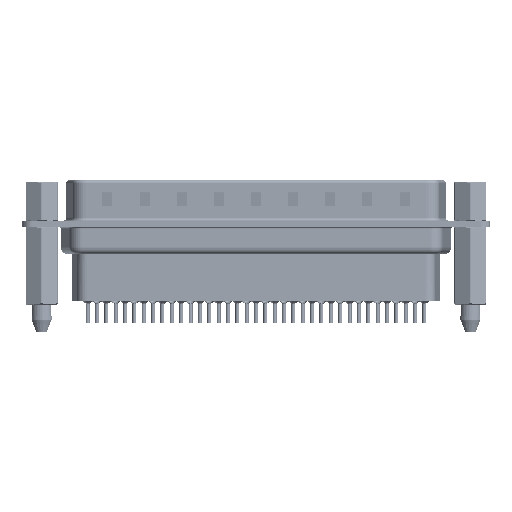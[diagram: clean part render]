
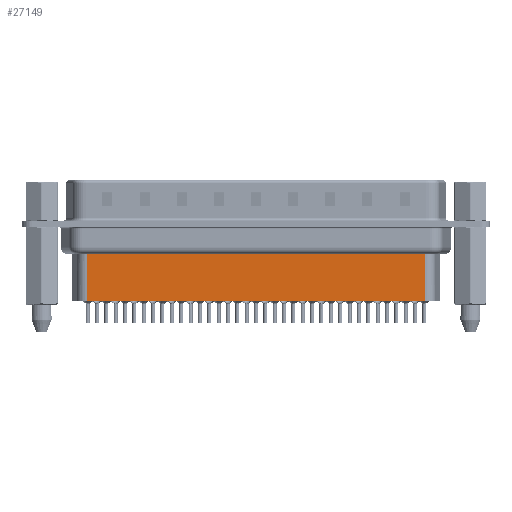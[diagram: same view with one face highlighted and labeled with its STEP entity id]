
A CAD part, front view. The second image highlights one B-rep face of the part: STEP entity #27149.
In plain terms, the highlighted planar face has unit normal (0, -1, 0).
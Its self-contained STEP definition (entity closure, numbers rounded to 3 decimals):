
#1149 = VECTOR ( 'NONE', #17048, 1000. ) ;
#1164 = EDGE_CURVE ( 'NONE', #26078, #18752, #14244, .T. ) ;
#1530 = CARTESIAN_POINT ( 'NONE',  ( 6.459, -3.5, -4.097 ) ) ;
#1653 = DIRECTION ( 'NONE',  ( -1., 0., 0. ) ) ;
#2057 = LINE ( 'NONE', #8477, #1149 ) ;
#3252 = CARTESIAN_POINT ( 'NONE',  ( 6.706, -3.5, -3.1 ) ) ;
#5884 = ORIENTED_EDGE ( 'NONE', *, *, #16960, .F. ) ;
#6689 = VECTOR ( 'NONE', #30666, 1000. ) ;
#8477 = CARTESIAN_POINT ( 'NONE',  ( 6.706, -3.5, -11.45 ) ) ;
#9018 = PLANE ( 'NONE',  #17963 ) ;
#9778 = VECTOR ( 'NONE', #1653, 1000. ) ;
#11886 = DIRECTION ( 'NONE',  ( 0., -1., 0. ) ) ;
#11914 = CARTESIAN_POINT ( 'NONE',  ( 6.706, -3.5, -11.45 ) ) ;
#12698 = FACE_OUTER_BOUND ( 'NONE', #29998, .T. ) ;
#14244 = LINE ( 'NONE', #29118, #6689 ) ;
#14692 = DIRECTION ( 'NONE',  ( 0., 0., -1. ) ) ;
#15475 = CARTESIAN_POINT ( 'NONE',  ( 56.794, -3.5, -11.45 ) ) ;
#16960 = EDGE_CURVE ( 'NONE', #18752, #26622, #2057, .T. ) ;
#17048 = DIRECTION ( 'NONE',  ( -1., 0., 0. ) ) ;
#17963 = AXIS2_PLACEMENT_3D ( 'NONE', #31549, #11886, #31799 ) ;
#18752 = VERTEX_POINT ( 'NONE', #15475 ) ;
#23432 = EDGE_CURVE ( 'NONE', #26078, #28002, #32514, .T. ) ;
#24513 = EDGE_CURVE ( 'NONE', #28002, #26622, #29343, .T. ) ;
#25743 = VECTOR ( 'NONE', #14692, 1000. ) ;
#26078 = VERTEX_POINT ( 'NONE', #35486 ) ;
#26622 = VERTEX_POINT ( 'NONE', #11914 ) ;
#27149 = ADVANCED_FACE ( 'NONE', ( #12698 ), #9018, .T. ) ;
#27735 = ORIENTED_EDGE ( 'NONE', *, *, #23432, .T. ) ;
#28002 = VERTEX_POINT ( 'NONE', #31839 ) ;
#29118 = CARTESIAN_POINT ( 'NONE',  ( 56.794, -3.5, -3.1 ) ) ;
#29343 = LINE ( 'NONE', #3252, #25743 ) ;
#29998 = EDGE_LOOP ( 'NONE', ( #36443, #27735, #33693, #5884 ) ) ;
#30666 = DIRECTION ( 'NONE',  ( 0., 0., -1. ) ) ;
#31549 = CARTESIAN_POINT ( 'NONE',  ( 6.706, -3.5, -3.1 ) ) ;
#31799 = DIRECTION ( 'NONE',  ( 1., 0., 0. ) ) ;
#31839 = CARTESIAN_POINT ( 'NONE',  ( 6.706, -3.5, -4.097 ) ) ;
#32514 = LINE ( 'NONE', #1530, #9778 ) ;
#33693 = ORIENTED_EDGE ( 'NONE', *, *, #24513, .T. ) ;
#35486 = CARTESIAN_POINT ( 'NONE',  ( 56.794, -3.5, -4.097 ) ) ;
#36443 = ORIENTED_EDGE ( 'NONE', *, *, #1164, .F. ) ;
